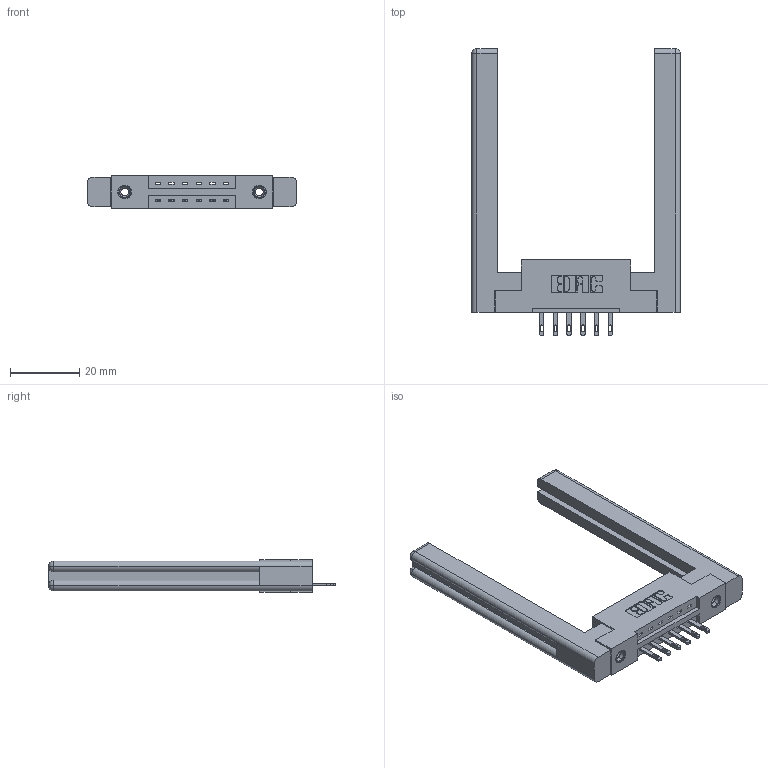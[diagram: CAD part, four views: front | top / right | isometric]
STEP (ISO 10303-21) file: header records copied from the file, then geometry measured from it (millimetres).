
FILE_DESCRIPTION (( 'STEP AP203' ), '1' );
FILE_NAME ('337-006-500-158.STEP', '2019-09-27T16:02:44', ( '' ), ( '' ), 'SwSTEP 2.0', 'SolidWorks 2016', '' );
FILE_SCHEMA (( 'CONFIG_CONTROL_DESIGN' ));
Length unit declared in the file: inch
Products named in the file (5): 337 Part_Flush Mounting Lugs - 0.156 Dia-TI; 307-220-058; 345-292-001_345-293-100; 345-250-001_345-250-001-102; 337-006-500-158
Assembly tree (11 placements, depth 2):
  337-006-500-158
    337 Part_Flush Mounting Lugs - 0.156 Dia-TI
    345-292-001_345-293-100  x6
    345-250-001_345-250-001-102  x2
    307-220-058  x2
Bounding box: 60.4 x 82.94 x 9.4 mm (x, y, z)
Volume: 12993.1 mm3; surface area: 11052.6 mm2
Topology: 11 solids, 11 shells, 604 faces, 1745 edges, 1150 vertices
Faces by surface type: plane 394, cylinder 186, cone 12, torus 12
Entity records: 11680 total; most frequent: CARTESIAN_POINT 2031, ORIENTED_EDGE 1912, DIRECTION 1804, EDGE_CURVE 956, LINE 776, VECTOR 776, VERTEX_POINT 630, AXIS2_PLACEMENT_3D 514
